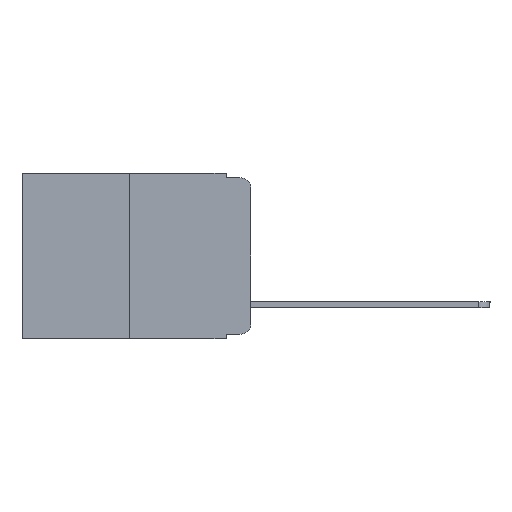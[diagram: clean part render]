
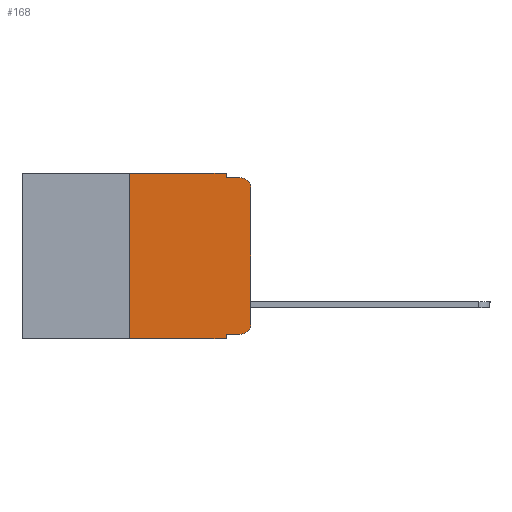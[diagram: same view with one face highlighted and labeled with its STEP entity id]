
A CAD part, left-side view. The second image highlights one B-rep face of the part: STEP entity #168.
In plain terms, the highlighted planar face has unit normal (-1, 0, 0).
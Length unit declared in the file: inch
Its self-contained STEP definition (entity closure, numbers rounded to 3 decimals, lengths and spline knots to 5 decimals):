
#21 = DIRECTION ( 'NONE',  ( 0., 0., 1. ) ) ;
#68 = EDGE_CURVE ( 'NONE', #4645, #83, #9476, .T. ) ;
#83 = VERTEX_POINT ( 'NONE', #18714 ) ;
#168 = ADVANCED_FACE ( 'NONE', ( #15617 ), #7572, .F. ) ;
#385 = CARTESIAN_POINT ( 'NONE',  ( 0., 0.473, 0. ) ) ;
#467 = VERTEX_POINT ( 'NONE', #14025 ) ;
#779 = EDGE_CURVE ( 'NONE', #16162, #19918, #17980, .T. ) ;
#942 = EDGE_CURVE ( 'NONE', #12573, #19081, #17112, .T. ) ;
#1216 = EDGE_CURVE ( 'NONE', #8770, #5735, #13564, .T. ) ;
#1350 = CARTESIAN_POINT ( 'NONE',  ( 0., 0.473, 0. ) ) ;
#2117 = DIRECTION ( 'NONE',  ( 0., 0., -1. ) ) ;
#2123 = DIRECTION ( 'NONE',  ( 0., -1., 0. ) ) ;
#2368 = ORIENTED_EDGE ( 'NONE', *, *, #942, .T. ) ;
#2822 = CARTESIAN_POINT ( 'NONE',  ( 0., 0.051, -0.333 ) ) ;
#2920 = EDGE_CURVE ( 'NONE', #8770, #467, #19584, .T. ) ;
#3188 = CARTESIAN_POINT ( 'NONE',  ( 0., 0.051, -0.343 ) ) ;
#4182 = DIRECTION ( 'NONE',  ( 0., -1., 0. ) ) ;
#4504 = EDGE_CURVE ( 'NONE', #467, #19529, #14763, .T. ) ;
#4645 = VERTEX_POINT ( 'NONE', #11342 ) ;
#4772 = ORIENTED_EDGE ( 'NONE', *, *, #2920, .F. ) ;
#4976 = AXIS2_PLACEMENT_3D ( 'NONE', #5651, #12021, #2117 ) ;
#5150 = CARTESIAN_POINT ( 'NONE',  ( 0., 0.02, -0.01 ) ) ;
#5277 = CARTESIAN_POINT ( 'NONE',  ( 0., 0.25, -0.343 ) ) ;
#5534 = CARTESIAN_POINT ( 'NONE',  ( 0., 0.02, -0.313 ) ) ;
#5651 = CARTESIAN_POINT ( 'NONE',  ( 0., 0.02, -0.03 ) ) ;
#5701 = ORIENTED_EDGE ( 'NONE', *, *, #4504, .F. ) ;
#5735 = VERTEX_POINT ( 'NONE', #3188 ) ;
#5738 = VECTOR ( 'NONE', #8744, 39.37008 ) ;
#5792 = DIRECTION ( 'NONE',  ( 0., 0., -1. ) ) ;
#6933 = CIRCLE ( 'NONE', #18904, 0.02 ) ;
#6974 = CIRCLE ( 'NONE', #4976, 0.02 ) ;
#7115 = VECTOR ( 'NONE', #21, 39.37008 ) ;
#7215 = VECTOR ( 'NONE', #2123, 39.37008 ) ;
#7245 = ORIENTED_EDGE ( 'NONE', *, *, #779, .F. ) ;
#7572 = PLANE ( 'NONE',  #12815 ) ;
#8398 = CARTESIAN_POINT ( 'NONE',  ( 0., 0.051, -0.333 ) ) ;
#8720 = ORIENTED_EDGE ( 'NONE', *, *, #15276, .F. ) ;
#8744 = DIRECTION ( 'NONE',  ( 0., 0., 1. ) ) ;
#8770 = VERTEX_POINT ( 'NONE', #5277 ) ;
#8945 = EDGE_LOOP ( 'NONE', ( #19107, #12456, #7245, #8720, #5701, #4772, #12138, #18793, #2368, #15474 ) ) ;
#9196 = EDGE_CURVE ( 'NONE', #83, #19918, #6974, .T. ) ;
#9476 = LINE ( 'NONE', #15852, #7115 ) ;
#10938 = VECTOR ( 'NONE', #5792, 39.37008 ) ;
#11342 = CARTESIAN_POINT ( 'NONE',  ( 0., 0., -0.313 ) ) ;
#11505 = LINE ( 'NONE', #16192, #15247 ) ;
#11708 = CARTESIAN_POINT ( 'NONE',  ( 0., 0.473, -0.343 ) ) ;
#11916 = DIRECTION ( 'NONE',  ( 0., 0., -1. ) ) ;
#12021 = DIRECTION ( 'NONE',  ( -1., 0., 0. ) ) ;
#12027 = CARTESIAN_POINT ( 'NONE',  ( 0., 0.051, -0.01 ) ) ;
#12138 = ORIENTED_EDGE ( 'NONE', *, *, #1216, .T. ) ;
#12293 = DIRECTION ( 'NONE',  ( 0., 0., -1. ) ) ;
#12456 = ORIENTED_EDGE ( 'NONE', *, *, #9196, .T. ) ;
#12573 = VERTEX_POINT ( 'NONE', #8398 ) ;
#12815 = AXIS2_PLACEMENT_3D ( 'NONE', #1350, #20374, #12293 ) ;
#13055 = EDGE_CURVE ( 'NONE', #12573, #5735, #11505, .T. ) ;
#13142 = EDGE_CURVE ( 'NONE', #19081, #4645, #6933, .T. ) ;
#13564 = LINE ( 'NONE', #11708, #15874 ) ;
#14025 = CARTESIAN_POINT ( 'NONE',  ( 0., 0.25, 0. ) ) ;
#14304 = CARTESIAN_POINT ( 'NONE',  ( 0., 0.051, -0.01 ) ) ;
#14763 = LINE ( 'NONE', #385, #16682 ) ;
#14829 = DIRECTION ( 'NONE',  ( 0., 0., -1. ) ) ;
#14898 = LINE ( 'NONE', #19970, #10938 ) ;
#15107 = CARTESIAN_POINT ( 'NONE',  ( 0., 0.25, 0. ) ) ;
#15247 = VECTOR ( 'NONE', #14829, 39.37008 ) ;
#15276 = EDGE_CURVE ( 'NONE', #19529, #16162, #14898, .T. ) ;
#15474 = ORIENTED_EDGE ( 'NONE', *, *, #13142, .T. ) ;
#15617 = FACE_OUTER_BOUND ( 'NONE', #8945, .T. ) ;
#15852 = CARTESIAN_POINT ( 'NONE',  ( 0., 0., 0. ) ) ;
#15874 = VECTOR ( 'NONE', #18133, 39.37008 ) ;
#16122 = DIRECTION ( 'NONE',  ( 0., -1., 0. ) ) ;
#16162 = VERTEX_POINT ( 'NONE', #14304 ) ;
#16192 = CARTESIAN_POINT ( 'NONE',  ( 0., 0.051, 0. ) ) ;
#16682 = VECTOR ( 'NONE', #16122, 39.37008 ) ;
#17112 = LINE ( 'NONE', #2822, #20538 ) ;
#17980 = LINE ( 'NONE', #12027, #7215 ) ;
#18036 = CARTESIAN_POINT ( 'NONE',  ( 0., 0.02, -0.333 ) ) ;
#18133 = DIRECTION ( 'NONE',  ( 0., -1., 0. ) ) ;
#18714 = CARTESIAN_POINT ( 'NONE',  ( 0., 0., -0.03 ) ) ;
#18793 = ORIENTED_EDGE ( 'NONE', *, *, #13055, .F. ) ;
#18904 = AXIS2_PLACEMENT_3D ( 'NONE', #5534, #19710, #11916 ) ;
#19081 = VERTEX_POINT ( 'NONE', #18036 ) ;
#19107 = ORIENTED_EDGE ( 'NONE', *, *, #68, .T. ) ;
#19446 = CARTESIAN_POINT ( 'NONE',  ( 0., 0.051, 0. ) ) ;
#19529 = VERTEX_POINT ( 'NONE', #19446 ) ;
#19584 = LINE ( 'NONE', #15107, #5738 ) ;
#19710 = DIRECTION ( 'NONE',  ( -1., 0., 0. ) ) ;
#19918 = VERTEX_POINT ( 'NONE', #5150 ) ;
#19970 = CARTESIAN_POINT ( 'NONE',  ( 0., 0.051, 0. ) ) ;
#20374 = DIRECTION ( 'NONE',  ( 1., 0., 0. ) ) ;
#20538 = VECTOR ( 'NONE', #4182, 39.37008 ) ;
